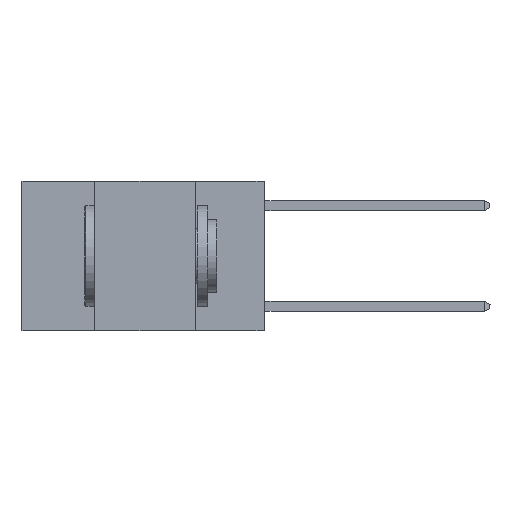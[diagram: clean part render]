
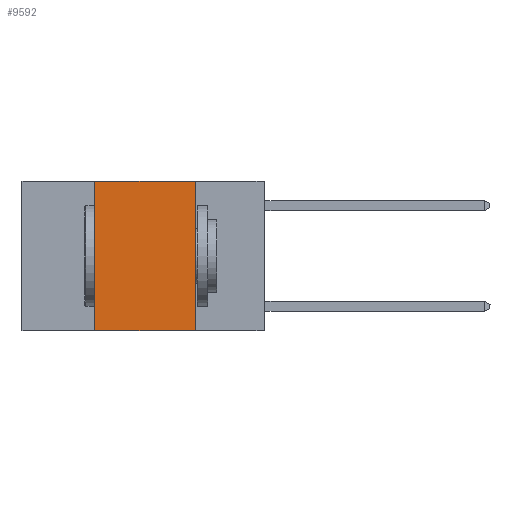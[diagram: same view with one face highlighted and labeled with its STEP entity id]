
A CAD part, left-side view. The second image highlights one B-rep face of the part: STEP entity #9592.
In plain terms, the highlighted planar face has unit normal (-1, 0, 0).
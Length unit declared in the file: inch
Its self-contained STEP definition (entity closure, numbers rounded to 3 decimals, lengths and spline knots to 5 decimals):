
#10 = VECTOR ( 'NONE', #12057, 39.37008 ) ;
#132 = ORIENTED_EDGE ( 'NONE', *, *, #10372, .T. ) ;
#1630 = PLANE ( 'NONE',  #22696 ) ;
#1960 = DIRECTION ( 'NONE',  ( 0., -1., 0. ) ) ;
#1966 = EDGE_CURVE ( 'NONE', #20844, #8409, #13411, .T. ) ;
#2248 = EDGE_CURVE ( 'NONE', #8409, #4341, #22592, .T. ) ;
#3552 = DIRECTION ( 'NONE',  ( 1., 0., 0. ) ) ;
#4341 = VERTEX_POINT ( 'NONE', #17024 ) ;
#4619 = FACE_OUTER_BOUND ( 'NONE', #18550, .T. ) ;
#4909 = ORIENTED_EDGE ( 'NONE', *, *, #2248, .F. ) ;
#7445 = VECTOR ( 'NONE', #8673, 39.37008 ) ;
#8075 = DIRECTION ( 'NONE',  ( 0., -1., 0. ) ) ;
#8409 = VERTEX_POINT ( 'NONE', #21201 ) ;
#8673 = DIRECTION ( 'NONE',  ( 0., 0., -1. ) ) ;
#9581 = LINE ( 'NONE', #23416, #10 ) ;
#9592 = ADVANCED_FACE ( 'NONE', ( #4619 ), #1630, .F. ) ;
#10372 = EDGE_CURVE ( 'NONE', #15011, #4341, #21488, .T. ) ;
#12057 = DIRECTION ( 'NONE',  ( 0., 0., 1. ) ) ;
#12498 = EDGE_CURVE ( 'NONE', #15011, #20844, #9581, .T. ) ;
#13177 = CARTESIAN_POINT ( 'NONE',  ( 0., 0.42, -0.37 ) ) ;
#13381 = CARTESIAN_POINT ( 'NONE',  ( 0., 0.6, -0.37 ) ) ;
#13411 = LINE ( 'NONE', #19453, #18447 ) ;
#14475 = CARTESIAN_POINT ( 'NONE',  ( 0., 0.17, 0. ) ) ;
#14940 = CARTESIAN_POINT ( 'NONE',  ( 0., 0.6, 0. ) ) ;
#15011 = VERTEX_POINT ( 'NONE', #13177 ) ;
#16443 = VECTOR ( 'NONE', #1960, 39.37008 ) ;
#16551 = CARTESIAN_POINT ( 'NONE',  ( 0., 0.42, 0. ) ) ;
#16846 = DIRECTION ( 'NONE',  ( 0., 0., -1. ) ) ;
#17024 = CARTESIAN_POINT ( 'NONE',  ( 0., 0.17, -0.37 ) ) ;
#18447 = VECTOR ( 'NONE', #8075, 39.37008 ) ;
#18550 = EDGE_LOOP ( 'NONE', ( #4909, #23052, #19180, #132 ) ) ;
#19180 = ORIENTED_EDGE ( 'NONE', *, *, #12498, .F. ) ;
#19453 = CARTESIAN_POINT ( 'NONE',  ( 0., 0.6, 0. ) ) ;
#20844 = VERTEX_POINT ( 'NONE', #16551 ) ;
#21201 = CARTESIAN_POINT ( 'NONE',  ( 0., 0.17, 0. ) ) ;
#21488 = LINE ( 'NONE', #13381, #16443 ) ;
#22592 = LINE ( 'NONE', #14475, #7445 ) ;
#22696 = AXIS2_PLACEMENT_3D ( 'NONE', #14940, #3552, #16846 ) ;
#23052 = ORIENTED_EDGE ( 'NONE', *, *, #1966, .F. ) ;
#23416 = CARTESIAN_POINT ( 'NONE',  ( 0., 0.42, 0. ) ) ;
